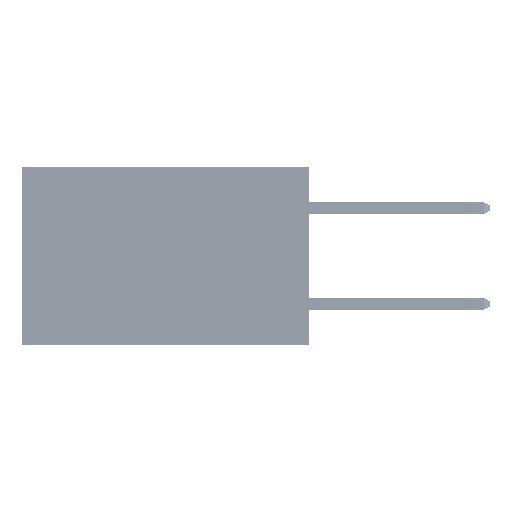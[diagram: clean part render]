
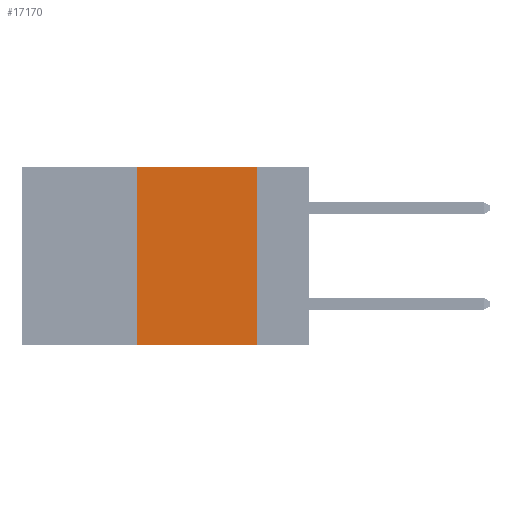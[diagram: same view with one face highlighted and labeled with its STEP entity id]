
A CAD part, left-side view. The second image highlights one B-rep face of the part: STEP entity #17170.
In plain terms, the highlighted planar face has unit normal (-1, 0, 0).
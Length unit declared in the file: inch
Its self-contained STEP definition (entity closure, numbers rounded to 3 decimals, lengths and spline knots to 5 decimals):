
#1403 = ORIENTED_EDGE ( 'NONE', *, *, #25934, .T. ) ;
#3233 = LINE ( 'NONE', #33827, #5777 ) ;
#3254 = EDGE_CURVE ( 'NONE', #18641, #7909, #10343, .T. ) ;
#5777 = VECTOR ( 'NONE', #29955, 39.37008 ) ;
#6707 = ORIENTED_EDGE ( 'NONE', *, *, #12998, .F. ) ;
#7909 = VERTEX_POINT ( 'NONE', #23714 ) ;
#10343 = LINE ( 'NONE', #38196, #20878 ) ;
#12998 = EDGE_CURVE ( 'NONE', #13045, #23992, #3233, .T. ) ;
#13045 = VERTEX_POINT ( 'NONE', #33659 ) ;
#14214 = DIRECTION ( 'NONE',  ( 0., 0., 1. ) ) ;
#14360 = ORIENTED_EDGE ( 'NONE', *, *, #17377, .F. ) ;
#15465 = CARTESIAN_POINT ( 'NONE',  ( 0., 0.6, 0. ) ) ;
#17170 = ADVANCED_FACE ( 'NONE', ( #31038 ), #38746, .F. ) ;
#17377 = EDGE_CURVE ( 'NONE', #7909, #13045, #41113, .T. ) ;
#18641 = VERTEX_POINT ( 'NONE', #23347 ) ;
#19085 = CARTESIAN_POINT ( 'NONE',  ( 0., 0.11, -0.37 ) ) ;
#19542 = VECTOR ( 'NONE', #19731, 39.37008 ) ;
#19731 = DIRECTION ( 'NONE',  ( 0., -1., 0. ) ) ;
#20878 = VECTOR ( 'NONE', #14214, 39.37008 ) ;
#22021 = AXIS2_PLACEMENT_3D ( 'NONE', #34300, #50577, #46666 ) ;
#22829 = EDGE_LOOP ( 'NONE', ( #6707, #14360, #31302, #1403 ) ) ;
#23347 = CARTESIAN_POINT ( 'NONE',  ( 0., 0.36, -0.37 ) ) ;
#23714 = CARTESIAN_POINT ( 'NONE',  ( 0., 0.36, 0. ) ) ;
#23992 = VERTEX_POINT ( 'NONE', #19085 ) ;
#25934 = EDGE_CURVE ( 'NONE', #18641, #23992, #51243, .T. ) ;
#29955 = DIRECTION ( 'NONE',  ( 0., 0., -1. ) ) ;
#31038 = FACE_OUTER_BOUND ( 'NONE', #22829, .T. ) ;
#31302 = ORIENTED_EDGE ( 'NONE', *, *, #3254, .F. ) ;
#33659 = CARTESIAN_POINT ( 'NONE',  ( 0., 0.11, 0. ) ) ;
#33827 = CARTESIAN_POINT ( 'NONE',  ( 0., 0.11, 0. ) ) ;
#34300 = CARTESIAN_POINT ( 'NONE',  ( 0., 0.6, 0. ) ) ;
#35923 = DIRECTION ( 'NONE',  ( 0., -1., 0. ) ) ;
#36461 = CARTESIAN_POINT ( 'NONE',  ( 0., 0.6, -0.37 ) ) ;
#38196 = CARTESIAN_POINT ( 'NONE',  ( 0., 0.36, 0. ) ) ;
#38746 = PLANE ( 'NONE',  #22021 ) ;
#40500 = VECTOR ( 'NONE', #35923, 39.37008 ) ;
#41113 = LINE ( 'NONE', #15465, #19542 ) ;
#46666 = DIRECTION ( 'NONE',  ( 0., 0., -1. ) ) ;
#50577 = DIRECTION ( 'NONE',  ( 1., 0., 0. ) ) ;
#51243 = LINE ( 'NONE', #36461, #40500 ) ;
